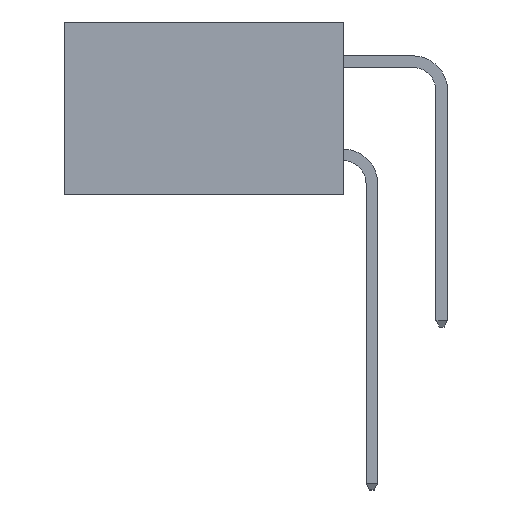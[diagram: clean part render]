
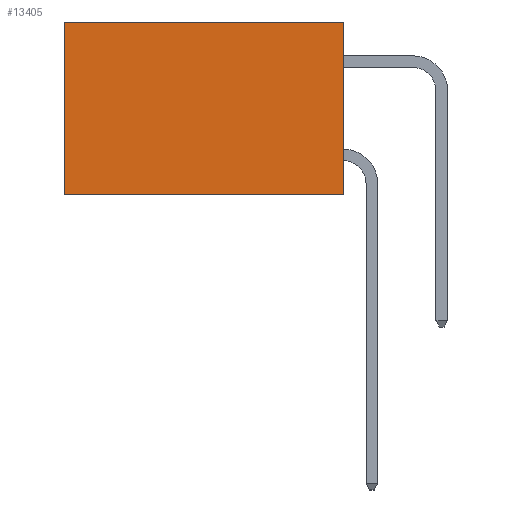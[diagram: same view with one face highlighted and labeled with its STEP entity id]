
A CAD part, left-side view. The second image highlights one B-rep face of the part: STEP entity #13405.
In plain terms, the highlighted planar face has unit normal (-1, 0, 0).
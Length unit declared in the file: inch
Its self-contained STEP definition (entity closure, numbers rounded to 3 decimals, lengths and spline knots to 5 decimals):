
#346 = VERTEX_POINT ( 'NONE', #13448 ) ;
#483 = VECTOR ( 'NONE', #11220, 39.37008 ) ;
#699 = ORIENTED_EDGE ( 'NONE', *, *, #10536, .F. ) ;
#976 = DIRECTION ( 'NONE',  ( 0., 0., -1. ) ) ;
#1170 = CARTESIAN_POINT ( 'NONE',  ( 0.2615, 0., -0.37 ) ) ;
#1398 = CARTESIAN_POINT ( 'NONE',  ( 0.2615, 0.6, -0.37 ) ) ;
#1518 = VECTOR ( 'NONE', #976, 39.37008 ) ;
#1785 = ORIENTED_EDGE ( 'NONE', *, *, #3362, .T. ) ;
#2885 = DIRECTION ( 'NONE',  ( 0., 0., -1. ) ) ;
#2949 = CARTESIAN_POINT ( 'NONE',  ( 0.2615, 0., -0.37 ) ) ;
#3091 = ORIENTED_EDGE ( 'NONE', *, *, #4465, .T. ) ;
#3121 = VERTEX_POINT ( 'NONE', #9994 ) ;
#3362 = EDGE_CURVE ( 'NONE', #8939, #346, #7875, .T. ) ;
#4231 = EDGE_CURVE ( 'NONE', #8939, #5759, #4809, .T. ) ;
#4465 = EDGE_CURVE ( 'NONE', #346, #3121, #4640, .T. ) ;
#4640 = LINE ( 'NONE', #1398, #1518 ) ;
#4809 = LINE ( 'NONE', #2949, #13403 ) ;
#5759 = VERTEX_POINT ( 'NONE', #10424 ) ;
#5850 = DIRECTION ( 'NONE',  ( 0., 0., -1. ) ) ;
#6366 = FACE_OUTER_BOUND ( 'NONE', #12358, .T. ) ;
#6967 = AXIS2_PLACEMENT_3D ( 'NONE', #1170, #12576, #5850 ) ;
#7509 = VECTOR ( 'NONE', #8429, 39.37008 ) ;
#7875 = LINE ( 'NONE', #8837, #7509 ) ;
#8429 = DIRECTION ( 'NONE',  ( 0., 1., 0. ) ) ;
#8837 = CARTESIAN_POINT ( 'NONE',  ( 0.2615, 0., 0. ) ) ;
#8939 = VERTEX_POINT ( 'NONE', #13911 ) ;
#9659 = LINE ( 'NONE', #10104, #483 ) ;
#9994 = CARTESIAN_POINT ( 'NONE',  ( 0.2615, 0.6, -0.37 ) ) ;
#10104 = CARTESIAN_POINT ( 'NONE',  ( 0.2615, 0., -0.37 ) ) ;
#10424 = CARTESIAN_POINT ( 'NONE',  ( 0.2615, 0., -0.37 ) ) ;
#10536 = EDGE_CURVE ( 'NONE', #5759, #3121, #9659, .T. ) ;
#11220 = DIRECTION ( 'NONE',  ( 0., 1., 0. ) ) ;
#11435 = PLANE ( 'NONE',  #6967 ) ;
#12358 = EDGE_LOOP ( 'NONE', ( #3091, #699, #14554, #1785 ) ) ;
#12576 = DIRECTION ( 'NONE',  ( 1., 0., 0. ) ) ;
#13403 = VECTOR ( 'NONE', #2885, 39.37008 ) ;
#13405 = ADVANCED_FACE ( 'NONE', ( #6366 ), #11435, .F. ) ;
#13448 = CARTESIAN_POINT ( 'NONE',  ( 0.2615, 0.6, 0. ) ) ;
#13911 = CARTESIAN_POINT ( 'NONE',  ( 0.2615, 0., 0. ) ) ;
#14554 = ORIENTED_EDGE ( 'NONE', *, *, #4231, .F. ) ;
